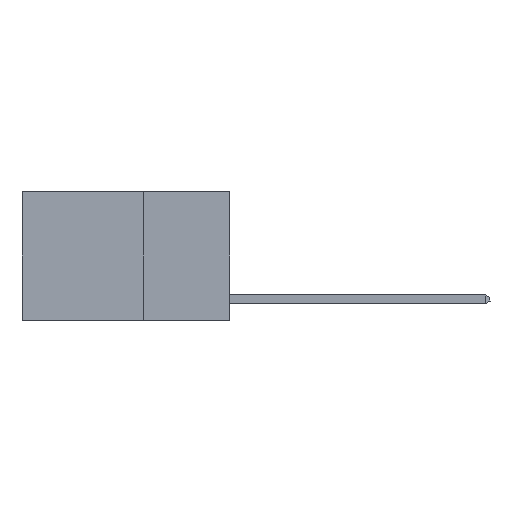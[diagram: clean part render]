
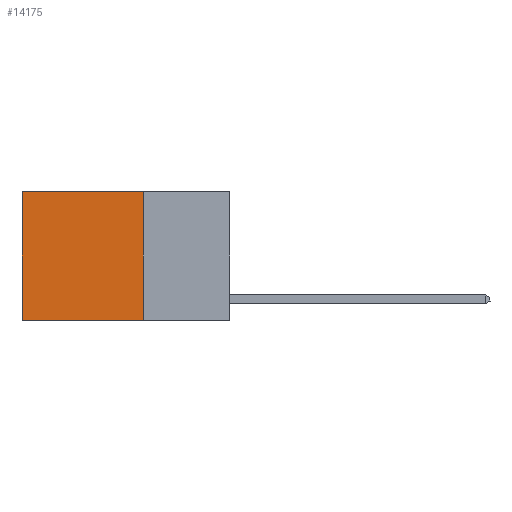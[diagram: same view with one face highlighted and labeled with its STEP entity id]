
A CAD part, left-side view. The second image highlights one B-rep face of the part: STEP entity #14175.
In plain terms, the highlighted planar face has unit normal (-1, 0, 0).
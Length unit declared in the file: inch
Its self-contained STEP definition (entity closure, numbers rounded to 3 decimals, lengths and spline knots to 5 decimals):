
#27 = VECTOR ( 'NONE', #11954, 39.37008 ) ;
#405 = LINE ( 'NONE', #6528, #7962 ) ;
#1538 = DIRECTION ( 'NONE',  ( 0., 0., -1. ) ) ;
#1702 = CARTESIAN_POINT ( 'NONE',  ( 0.2625, 0.25, -0.37 ) ) ;
#1880 = ORIENTED_EDGE ( 'NONE', *, *, #4229, .T. ) ;
#1905 = DIRECTION ( 'NONE',  ( 0., 0., -1. ) ) ;
#1993 = CARTESIAN_POINT ( 'NONE',  ( 0.2625, 0.25, 0. ) ) ;
#3207 = LINE ( 'NONE', #1993, #3292 ) ;
#3275 = VERTEX_POINT ( 'NONE', #4502 ) ;
#3292 = VECTOR ( 'NONE', #5294, 39.37008 ) ;
#4033 = CARTESIAN_POINT ( 'NONE',  ( 0.2625, 0.25, 0. ) ) ;
#4229 = EDGE_CURVE ( 'NONE', #5584, #10321, #12629, .T. ) ;
#4350 = EDGE_CURVE ( 'NONE', #9327, #10321, #6160, .T. ) ;
#4502 = CARTESIAN_POINT ( 'NONE',  ( 0.2625, 0.25, 0. ) ) ;
#4929 = DIRECTION ( 'NONE',  ( 0., 1., 0. ) ) ;
#5294 = DIRECTION ( 'NONE',  ( 0., 1., 0. ) ) ;
#5584 = VERTEX_POINT ( 'NONE', #6725 ) ;
#6160 = LINE ( 'NONE', #12091, #11547 ) ;
#6420 = FACE_OUTER_BOUND ( 'NONE', #7327, .T. ) ;
#6528 = CARTESIAN_POINT ( 'NONE',  ( 0.2625, 0.25, 0. ) ) ;
#6725 = CARTESIAN_POINT ( 'NONE',  ( 0.2625, 0.6, 0. ) ) ;
#6880 = ORIENTED_EDGE ( 'NONE', *, *, #13737, .T. ) ;
#6976 = ORIENTED_EDGE ( 'NONE', *, *, #10562, .F. ) ;
#7327 = EDGE_LOOP ( 'NONE', ( #1880, #11350, #6976, #6880 ) ) ;
#7962 = VECTOR ( 'NONE', #1538, 39.37008 ) ;
#8478 = CARTESIAN_POINT ( 'NONE',  ( 0.2625, 0.6, 0. ) ) ;
#9327 = VERTEX_POINT ( 'NONE', #1702 ) ;
#9443 = AXIS2_PLACEMENT_3D ( 'NONE', #4033, #14757, #1905 ) ;
#10321 = VERTEX_POINT ( 'NONE', #12684 ) ;
#10562 = EDGE_CURVE ( 'NONE', #3275, #9327, #405, .T. ) ;
#11350 = ORIENTED_EDGE ( 'NONE', *, *, #4350, .F. ) ;
#11547 = VECTOR ( 'NONE', #4929, 39.37008 ) ;
#11954 = DIRECTION ( 'NONE',  ( 0., 0., -1. ) ) ;
#12091 = CARTESIAN_POINT ( 'NONE',  ( 0.2625, 0.25, -0.37 ) ) ;
#12629 = LINE ( 'NONE', #8478, #27 ) ;
#12684 = CARTESIAN_POINT ( 'NONE',  ( 0.2625, 0.6, -0.37 ) ) ;
#13697 = PLANE ( 'NONE',  #9443 ) ;
#13737 = EDGE_CURVE ( 'NONE', #3275, #5584, #3207, .T. ) ;
#14175 = ADVANCED_FACE ( 'NONE', ( #6420 ), #13697, .F. ) ;
#14757 = DIRECTION ( 'NONE',  ( 1., 0., 0. ) ) ;
